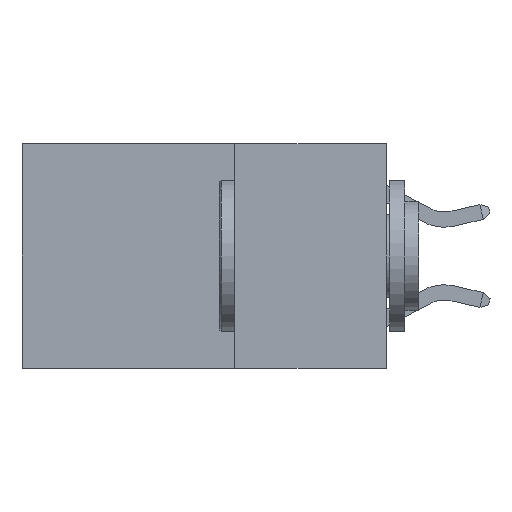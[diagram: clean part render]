
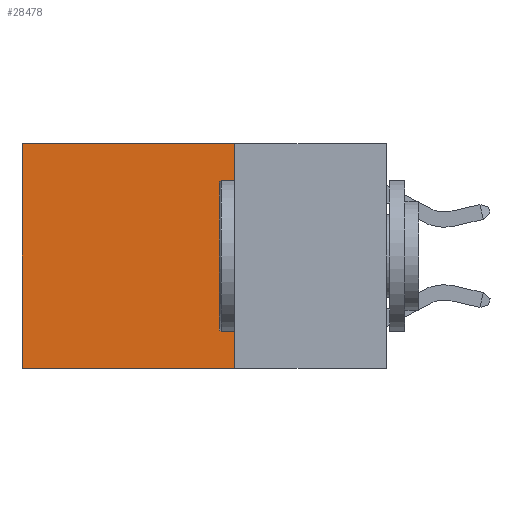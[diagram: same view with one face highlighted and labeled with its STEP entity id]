
A CAD part, left-side view. The second image highlights one B-rep face of the part: STEP entity #28478.
In plain terms, the highlighted planar face has unit normal (-1, 0, 0).
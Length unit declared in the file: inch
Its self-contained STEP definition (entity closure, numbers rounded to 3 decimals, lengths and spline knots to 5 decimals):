
#76 = CARTESIAN_POINT ( 'NONE',  ( 0.2625, 0.6, -0.37 ) ) ;
#352 = ORIENTED_EDGE ( 'NONE', *, *, #13358, .F. ) ;
#947 = DIRECTION ( 'NONE',  ( 0., 0., -1. ) ) ;
#1572 = VECTOR ( 'NONE', #11961, 39.37008 ) ;
#2091 = VECTOR ( 'NONE', #947, 39.37008 ) ;
#7328 = VECTOR ( 'NONE', #11219, 39.37008 ) ;
#7613 = PLANE ( 'NONE',  #20127 ) ;
#7871 = CARTESIAN_POINT ( 'NONE',  ( 0.2625, 0.6, 0. ) ) ;
#7982 = VERTEX_POINT ( 'NONE', #27188 ) ;
#8170 = CARTESIAN_POINT ( 'NONE',  ( 0.2625, 0.25, -0.37 ) ) ;
#10029 = CARTESIAN_POINT ( 'NONE',  ( 0.2625, 0.25, 0. ) ) ;
#11125 = CARTESIAN_POINT ( 'NONE',  ( 0.2625, 0.25, 0. ) ) ;
#11219 = DIRECTION ( 'NONE',  ( 0., 0., -1. ) ) ;
#11961 = DIRECTION ( 'NONE',  ( 0., 1., 0. ) ) ;
#12232 = FACE_OUTER_BOUND ( 'NONE', #22841, .T. ) ;
#12336 = DIRECTION ( 'NONE',  ( 0., 0., -1. ) ) ;
#12862 = ORIENTED_EDGE ( 'NONE', *, *, #20774, .T. ) ;
#13358 = EDGE_CURVE ( 'NONE', #7982, #25735, #26048, .T. ) ;
#13811 = LINE ( 'NONE', #23161, #1572 ) ;
#14136 = VERTEX_POINT ( 'NONE', #7871 ) ;
#14514 = CARTESIAN_POINT ( 'NONE',  ( 0.2625, 0.25, 0. ) ) ;
#15018 = VECTOR ( 'NONE', #25754, 39.37008 ) ;
#16938 = CARTESIAN_POINT ( 'NONE',  ( 0.2625, 0.6, 0. ) ) ;
#18317 = ORIENTED_EDGE ( 'NONE', *, *, #20851, .T. ) ;
#18637 = ORIENTED_EDGE ( 'NONE', *, *, #26174, .F. ) ;
#19582 = LINE ( 'NONE', #16938, #2091 ) ;
#20127 = AXIS2_PLACEMENT_3D ( 'NONE', #10029, #25776, #12336 ) ;
#20774 = EDGE_CURVE ( 'NONE', #7982, #14136, #20982, .T. ) ;
#20851 = EDGE_CURVE ( 'NONE', #14136, #21913, #19582, .T. ) ;
#20982 = LINE ( 'NONE', #14514, #15018 ) ;
#21913 = VERTEX_POINT ( 'NONE', #76 ) ;
#22841 = EDGE_LOOP ( 'NONE', ( #18317, #18637, #352, #12862 ) ) ;
#23161 = CARTESIAN_POINT ( 'NONE',  ( 0.2625, 0.25, -0.37 ) ) ;
#25735 = VERTEX_POINT ( 'NONE', #8170 ) ;
#25754 = DIRECTION ( 'NONE',  ( 0., 1., 0. ) ) ;
#25776 = DIRECTION ( 'NONE',  ( 1., 0., 0. ) ) ;
#26048 = LINE ( 'NONE', #11125, #7328 ) ;
#26174 = EDGE_CURVE ( 'NONE', #25735, #21913, #13811, .T. ) ;
#27188 = CARTESIAN_POINT ( 'NONE',  ( 0.2625, 0.25, 0. ) ) ;
#28478 = ADVANCED_FACE ( 'NONE', ( #12232 ), #7613, .F. ) ;
